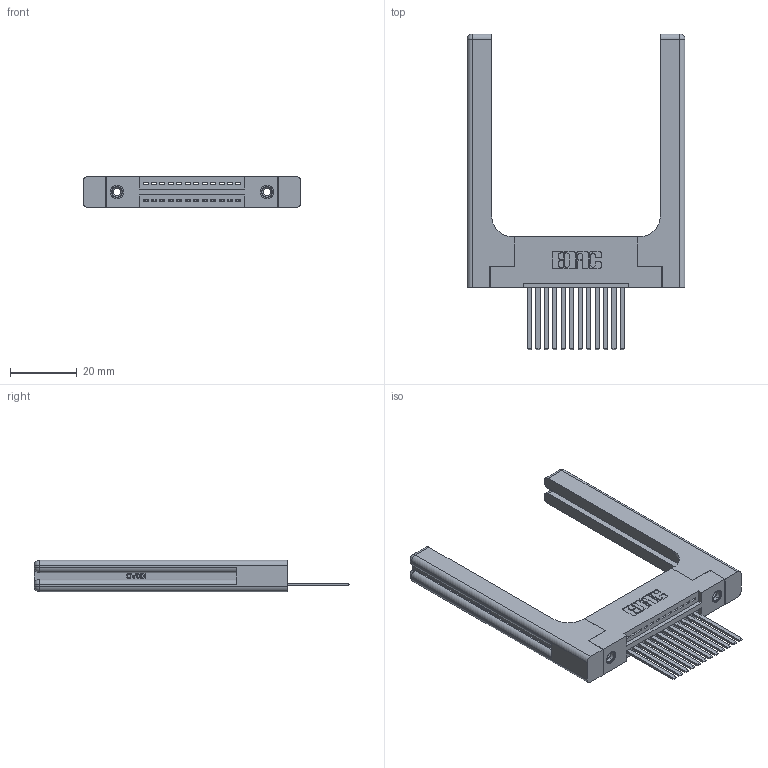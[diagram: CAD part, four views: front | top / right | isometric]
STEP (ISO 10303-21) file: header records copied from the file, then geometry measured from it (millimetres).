
FILE_DESCRIPTION (( 'STEP AP203' ), '1' );
FILE_NAME ('395-012-544-158.STEP', '2019-10-16T01:30:23', ( '' ), ( '' ), 'SwSTEP 2.0', 'SolidWorks 2016', '' );
FILE_SCHEMA (( 'CONFIG_CONTROL_DESIGN' ));
Length unit declared in the file: inch
Products named in the file (5): 395-012-544-158; 345 Part_Flush Mounting Lugs - 0.156 Dia-TH; 345-250-001_345-250-001-102; 345-220-058_345-220-058; 345-292-001_345-293-144
Assembly tree (17 placements, depth 2):
  395-012-544-158
    345 Part_Flush Mounting Lugs - 0.156 Dia-TH
    345-292-001_345-293-144  x12
    345-250-001_345-250-001-102  x2
    345-220-058_345-220-058  x2
Bounding box: 65.51 x 94.92 x 9.4 mm (x, y, z)
Volume: 14620.1 mm3; surface area: 13441.5 mm2
Topology: 17 solids, 17 shells, 1006 faces, 2903 edges, 1898 vertices
Faces by surface type: plane 660, cylinder 286, bspline 36, cone 12, sphere 8, torus 4
Entity records: 18068 total; most frequent: CARTESIAN_POINT 4101, ORIENTED_EDGE 2844, DIRECTION 2570, EDGE_CURVE 1422, VECTOR 1154, LINE 1154, VERTEX_POINT 938, AXIS2_PLACEMENT_3D 708
